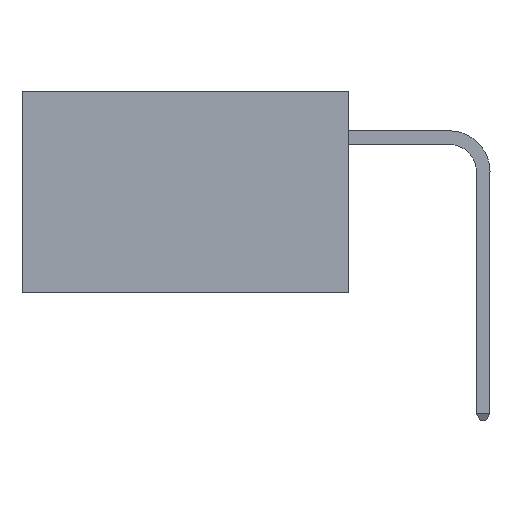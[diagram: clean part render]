
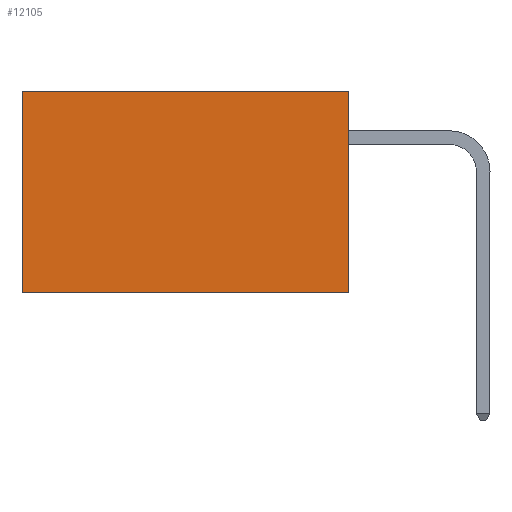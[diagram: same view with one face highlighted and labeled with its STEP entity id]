
A CAD part, left-side view. The second image highlights one B-rep face of the part: STEP entity #12105.
In plain terms, the highlighted planar face has unit normal (-1, 0, 0).
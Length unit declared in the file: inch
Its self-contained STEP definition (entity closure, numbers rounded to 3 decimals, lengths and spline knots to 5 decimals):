
#250 = EDGE_CURVE ( 'NONE', #8221, #6990, #6965, .T. ) ;
#1169 = CARTESIAN_POINT ( 'NONE',  ( 0.2875, 0., -0.37 ) ) ;
#1884 = AXIS2_PLACEMENT_3D ( 'NONE', #13421, #6905, #6953 ) ;
#2512 = FACE_OUTER_BOUND ( 'NONE', #11559, .T. ) ;
#2689 = LINE ( 'NONE', #10460, #13900 ) ;
#2879 = ORIENTED_EDGE ( 'NONE', *, *, #250, .F. ) ;
#3519 = CARTESIAN_POINT ( 'NONE',  ( 0.2875, 0.6, -0.37 ) ) ;
#4038 = ORIENTED_EDGE ( 'NONE', *, *, #14024, .F. ) ;
#4570 = LINE ( 'NONE', #12239, #10498 ) ;
#4765 = CARTESIAN_POINT ( 'NONE',  ( 0.2875, 0., -0.37 ) ) ;
#5247 = VECTOR ( 'NONE', #8801, 39.37008 ) ;
#5724 = LINE ( 'NONE', #6135, #14016 ) ;
#6135 = CARTESIAN_POINT ( 'NONE',  ( 0.2875, 0., 0. ) ) ;
#6905 = DIRECTION ( 'NONE',  ( 1., 0., 0. ) ) ;
#6953 = DIRECTION ( 'NONE',  ( 0., 0., -1. ) ) ;
#6965 = LINE ( 'NONE', #1169, #5247 ) ;
#6990 = VERTEX_POINT ( 'NONE', #3519 ) ;
#7222 = DIRECTION ( 'NONE',  ( 0., 0., -1. ) ) ;
#7572 = DIRECTION ( 'NONE',  ( 0., 1., 0. ) ) ;
#8221 = VERTEX_POINT ( 'NONE', #4765 ) ;
#8480 = VERTEX_POINT ( 'NONE', #9615 ) ;
#8801 = DIRECTION ( 'NONE',  ( 0., 1., 0. ) ) ;
#9255 = DIRECTION ( 'NONE',  ( 0., 0., -1. ) ) ;
#9615 = CARTESIAN_POINT ( 'NONE',  ( 0.2875, 0.6, 0. ) ) ;
#9733 = ORIENTED_EDGE ( 'NONE', *, *, #10548, .T. ) ;
#10460 = CARTESIAN_POINT ( 'NONE',  ( 0.2875, 0.6, 0. ) ) ;
#10498 = VECTOR ( 'NONE', #7572, 39.37008 ) ;
#10548 = EDGE_CURVE ( 'NONE', #8480, #6990, #2689, .T. ) ;
#11559 = EDGE_LOOP ( 'NONE', ( #9733, #2879, #4038, #12439 ) ) ;
#11972 = EDGE_CURVE ( 'NONE', #12415, #8480, #4570, .T. ) ;
#12105 = ADVANCED_FACE ( 'NONE', ( #2512 ), #12332, .F. ) ;
#12239 = CARTESIAN_POINT ( 'NONE',  ( 0.2875, 0., 0. ) ) ;
#12332 = PLANE ( 'NONE',  #1884 ) ;
#12415 = VERTEX_POINT ( 'NONE', #12518 ) ;
#12439 = ORIENTED_EDGE ( 'NONE', *, *, #11972, .T. ) ;
#12518 = CARTESIAN_POINT ( 'NONE',  ( 0.2875, 0., 0. ) ) ;
#13421 = CARTESIAN_POINT ( 'NONE',  ( 0.2875, 0., 0. ) ) ;
#13900 = VECTOR ( 'NONE', #9255, 39.37008 ) ;
#14016 = VECTOR ( 'NONE', #7222, 39.37008 ) ;
#14024 = EDGE_CURVE ( 'NONE', #12415, #8221, #5724, .T. ) ;
